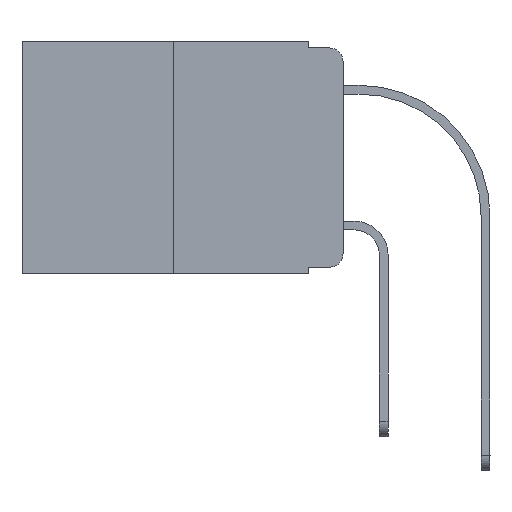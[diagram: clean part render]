
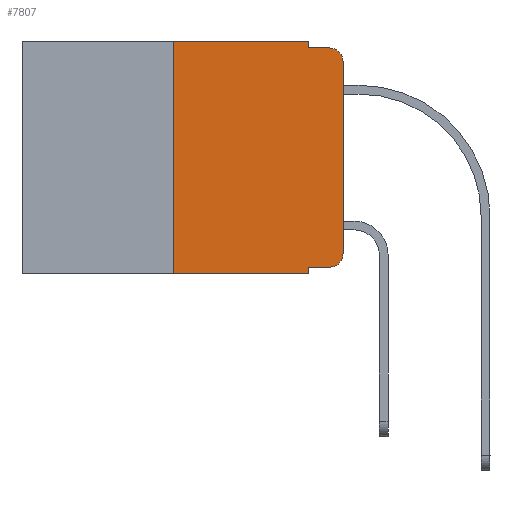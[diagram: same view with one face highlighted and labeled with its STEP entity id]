
A CAD part, left-side view. The second image highlights one B-rep face of the part: STEP entity #7807.
In plain terms, the highlighted planar face has unit normal (-1, 0, 0).
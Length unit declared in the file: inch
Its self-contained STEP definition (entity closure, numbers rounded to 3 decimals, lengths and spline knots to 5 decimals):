
#37 = ORIENTED_EDGE ( 'NONE', *, *, #6813, .T. ) ;
#246 = LINE ( 'NONE', #8362, #12510 ) ;
#449 = CARTESIAN_POINT ( 'NONE',  ( 0., 0.051, 0. ) ) ;
#594 = VERTEX_POINT ( 'NONE', #4164 ) ;
#1259 = EDGE_LOOP ( 'NONE', ( #5098, #37, #8983, #12429, #9052, #11608, #8267, #3702, #7303, #11876 ) ) ;
#1326 = CARTESIAN_POINT ( 'NONE',  ( 0., 0.25, -0.343 ) ) ;
#1343 = PLANE ( 'NONE',  #12879 ) ;
#1401 = VECTOR ( 'NONE', #5653, 39.37008 ) ;
#1636 = DIRECTION ( 'NONE',  ( 1., 0., 0. ) ) ;
#1637 = VERTEX_POINT ( 'NONE', #1326 ) ;
#1652 = CIRCLE ( 'NONE', #4031, 0.02 ) ;
#1846 = DIRECTION ( 'NONE',  ( 0., 0., -1. ) ) ;
#2020 = VERTEX_POINT ( 'NONE', #7942 ) ;
#2286 = CARTESIAN_POINT ( 'NONE',  ( 0., 0.02, -0.03 ) ) ;
#2291 = VERTEX_POINT ( 'NONE', #12953 ) ;
#2593 = FACE_OUTER_BOUND ( 'NONE', #1259, .T. ) ;
#2639 = DIRECTION ( 'NONE',  ( 0., 0., 1. ) ) ;
#3050 = CARTESIAN_POINT ( 'NONE',  ( 0., 0.051, 0. ) ) ;
#3073 = VECTOR ( 'NONE', #11403, 39.37008 ) ;
#3563 = CIRCLE ( 'NONE', #8092, 0.02 ) ;
#3644 = CARTESIAN_POINT ( 'NONE',  ( 0., 0.473, 0. ) ) ;
#3685 = VECTOR ( 'NONE', #9219, 39.37008 ) ;
#3702 = ORIENTED_EDGE ( 'NONE', *, *, #11804, .F. ) ;
#3958 = DIRECTION ( 'NONE',  ( 0., 0., -1. ) ) ;
#4029 = DIRECTION ( 'NONE',  ( 0., -1., 0. ) ) ;
#4031 = AXIS2_PLACEMENT_3D ( 'NONE', #7666, #12255, #3958 ) ;
#4164 = CARTESIAN_POINT ( 'NONE',  ( 0., 0.051, -0.01 ) ) ;
#4457 = CARTESIAN_POINT ( 'NONE',  ( 0., 0.051, -0.01 ) ) ;
#5076 = CARTESIAN_POINT ( 'NONE',  ( 0., 0.02, -0.01 ) ) ;
#5098 = ORIENTED_EDGE ( 'NONE', *, *, #10894, .T. ) ;
#5205 = DIRECTION ( 'NONE',  ( 0., 0., -1. ) ) ;
#5301 = VERTEX_POINT ( 'NONE', #9030 ) ;
#5512 = VERTEX_POINT ( 'NONE', #449 ) ;
#5653 = DIRECTION ( 'NONE',  ( 0., -1., 0. ) ) ;
#5879 = DIRECTION ( 'NONE',  ( 0., -1., 0. ) ) ;
#6211 = VERTEX_POINT ( 'NONE', #11878 ) ;
#6258 = EDGE_CURVE ( 'NONE', #1637, #7622, #8524, .T. ) ;
#6379 = EDGE_CURVE ( 'NONE', #2020, #5301, #1652, .T. ) ;
#6495 = EDGE_CURVE ( 'NONE', #7078, #5512, #7818, .T. ) ;
#6813 = EDGE_CURVE ( 'NONE', #6211, #9168, #3563, .T. ) ;
#7078 = VERTEX_POINT ( 'NONE', #13709 ) ;
#7101 = CARTESIAN_POINT ( 'NONE',  ( 0., 0.25, 0. ) ) ;
#7303 = ORIENTED_EDGE ( 'NONE', *, *, #13550, .T. ) ;
#7622 = VERTEX_POINT ( 'NONE', #9729 ) ;
#7666 = CARTESIAN_POINT ( 'NONE',  ( 0., 0.02, -0.313 ) ) ;
#7726 = DIRECTION ( 'NONE',  ( 0., 0., -1. ) ) ;
#7807 = ADVANCED_FACE ( 'NONE', ( #2593 ), #1343, .F. ) ;
#7818 = LINE ( 'NONE', #12404, #1401 ) ;
#7884 = LINE ( 'NONE', #4457, #3073 ) ;
#7942 = CARTESIAN_POINT ( 'NONE',  ( 0., 0.02, -0.333 ) ) ;
#8075 = EDGE_CURVE ( 'NONE', #594, #9168, #7884, .T. ) ;
#8092 = AXIS2_PLACEMENT_3D ( 'NONE', #2286, #9981, #7726 ) ;
#8267 = ORIENTED_EDGE ( 'NONE', *, *, #6258, .T. ) ;
#8362 = CARTESIAN_POINT ( 'NONE',  ( 0., 0.051, -0.333 ) ) ;
#8524 = LINE ( 'NONE', #12028, #9272 ) ;
#8647 = CARTESIAN_POINT ( 'NONE',  ( 0., 0.051, 0. ) ) ;
#8983 = ORIENTED_EDGE ( 'NONE', *, *, #8075, .F. ) ;
#9030 = CARTESIAN_POINT ( 'NONE',  ( 0., 0., -0.313 ) ) ;
#9052 = ORIENTED_EDGE ( 'NONE', *, *, #6495, .F. ) ;
#9168 = VERTEX_POINT ( 'NONE', #5076 ) ;
#9219 = DIRECTION ( 'NONE',  ( 0., 0., 1. ) ) ;
#9272 = VECTOR ( 'NONE', #4029, 39.37008 ) ;
#9522 = LINE ( 'NONE', #12743, #12930 ) ;
#9692 = LINE ( 'NONE', #8647, #13654 ) ;
#9729 = CARTESIAN_POINT ( 'NONE',  ( 0., 0.051, -0.343 ) ) ;
#9821 = VECTOR ( 'NONE', #5205, 39.37008 ) ;
#9981 = DIRECTION ( 'NONE',  ( -1., 0., 0. ) ) ;
#10196 = EDGE_CURVE ( 'NONE', #5512, #594, #11047, .T. ) ;
#10672 = DIRECTION ( 'NONE',  ( 0., 0., -1. ) ) ;
#10894 = EDGE_CURVE ( 'NONE', #5301, #6211, #9522, .T. ) ;
#11047 = LINE ( 'NONE', #3050, #9821 ) ;
#11403 = DIRECTION ( 'NONE',  ( 0., -1., 0. ) ) ;
#11608 = ORIENTED_EDGE ( 'NONE', *, *, #14421, .F. ) ;
#11684 = LINE ( 'NONE', #7101, #3685 ) ;
#11804 = EDGE_CURVE ( 'NONE', #2291, #7622, #9692, .T. ) ;
#11876 = ORIENTED_EDGE ( 'NONE', *, *, #6379, .T. ) ;
#11878 = CARTESIAN_POINT ( 'NONE',  ( 0., 0., -0.03 ) ) ;
#12028 = CARTESIAN_POINT ( 'NONE',  ( 0., 0.473, -0.343 ) ) ;
#12255 = DIRECTION ( 'NONE',  ( -1., 0., 0. ) ) ;
#12404 = CARTESIAN_POINT ( 'NONE',  ( 0., 0.473, 0. ) ) ;
#12429 = ORIENTED_EDGE ( 'NONE', *, *, #10196, .F. ) ;
#12510 = VECTOR ( 'NONE', #5879, 39.37008 ) ;
#12743 = CARTESIAN_POINT ( 'NONE',  ( 0., 0., 0. ) ) ;
#12879 = AXIS2_PLACEMENT_3D ( 'NONE', #3644, #1636, #10672 ) ;
#12930 = VECTOR ( 'NONE', #2639, 39.37008 ) ;
#12953 = CARTESIAN_POINT ( 'NONE',  ( 0., 0.051, -0.333 ) ) ;
#13550 = EDGE_CURVE ( 'NONE', #2291, #2020, #246, .T. ) ;
#13654 = VECTOR ( 'NONE', #1846, 39.37008 ) ;
#13709 = CARTESIAN_POINT ( 'NONE',  ( 0., 0.25, 0. ) ) ;
#14421 = EDGE_CURVE ( 'NONE', #1637, #7078, #11684, .T. ) ;
